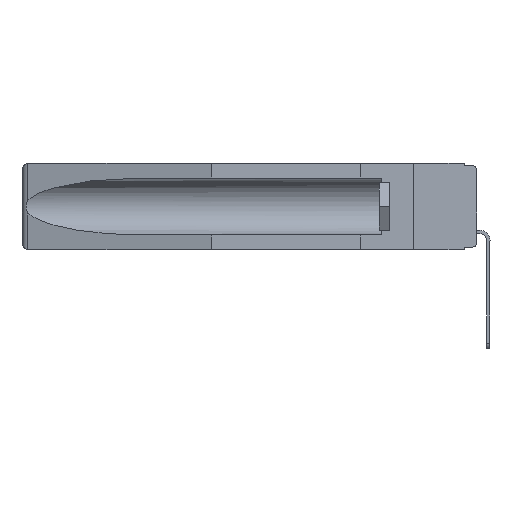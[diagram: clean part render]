
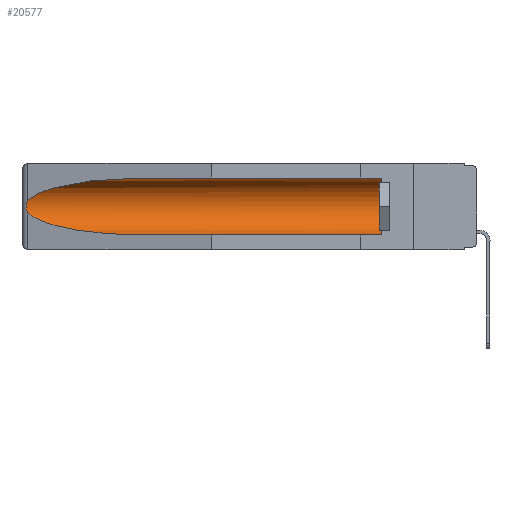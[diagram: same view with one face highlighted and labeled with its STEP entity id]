
A CAD part, left-side view. The second image highlights one B-rep face of the part: STEP entity #20577.
In plain terms, the highlighted cylindrical face has radius 2.857 mm (diameter 5.715 mm), a partial arc.
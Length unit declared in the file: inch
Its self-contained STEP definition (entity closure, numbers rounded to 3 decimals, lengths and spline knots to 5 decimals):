
#275 = CARTESIAN_POINT ( 'NONE',  ( 0.26537, 1.52718, -0.19328 ) ) ;
#886 = ORIENTED_EDGE ( 'NONE', *, *, #13939, .T. ) ;
#1474 = VECTOR ( 'NONE', #20221, 39.37008 ) ;
#1631 = CARTESIAN_POINT ( 'NONE',  ( 0.26537, 1.52718, -0.19328 ) ) ;
#1986 = VERTEX_POINT ( 'NONE', #13730 ) ;
#2005 = LINE ( 'NONE', #2962, #1474 ) ;
#2304 = FACE_OUTER_BOUND ( 'NONE', #18961, .T. ) ;
#2488 = DIRECTION ( 'NONE',  ( 0., 0., 1. ) ) ;
#2566 = CARTESIAN_POINT ( 'NONE',  ( 0.155, 0.126, -0.059 ) ) ;
#2868 = CARTESIAN_POINT ( 'NONE',  ( 0.155, 0.126, -0.284 ) ) ;
#2962 = CARTESIAN_POINT ( 'NONE',  ( 0.155, -0.30754, -0.284 ) ) ;
#3225 = CARTESIAN_POINT ( 'NONE',  ( 0.2673, 1.5327, -0.16383 ) ) ;
#4005 = VERTEX_POINT ( 'NONE', #9888 ) ;
#4371 = B_SPLINE_CURVE_WITH_KNOTS ( 'NONE', 3,
 ( #8322, #6607, #12025, #3225, #10225, #15482, #6770, #18825, #20487, #1631 ),
 .UNSPECIFIED., .F., .F.,
 ( 4, 2, 2, 2, 4 ),
 ( 0., 0.00029, 0.00058, 0.00087, 0.00117 ),
 .UNSPECIFIED. ) ;
#4438 = AXIS2_PLACEMENT_3D ( 'NONE', #12884, #14529, #2488 ) ;
#4991 = DIRECTION ( 'NONE',  ( 0., 1., 0. ) ) ;
#5295 = VERTEX_POINT ( 'NONE', #13356 ) ;
#5357 = CARTESIAN_POINT ( 'NONE',  ( 0.25451, 1.48313, -0.24835 ) ) ;
#5418 = CARTESIAN_POINT ( 'NONE',  ( 0.21114, 1.30732, -0.284 ) ) ;
#5749 =( BOUNDED_CURVE ( )  B_SPLINE_CURVE ( 3, ( #275, #5357, #5418, #10548 ),
 .UNSPECIFIED., .F., .F. ) 
 B_SPLINE_CURVE_WITH_KNOTS ( ( 4, 4 ),
 ( 0.1948, 1.5708 ),
 .UNSPECIFIED. ) 
 CURVE ( )  GEOMETRIC_REPRESENTATION_ITEM ( )  RATIONAL_B_SPLINE_CURVE ( ( 1., 0.848, 0.848, 1. ) ) 
 REPRESENTATION_ITEM ( '' )  );
#6581 = AXIS2_PLACEMENT_3D ( 'NONE', #17329, #21010, #17263 ) ;
#6607 = CARTESIAN_POINT ( 'NONE',  ( 0.26597, 1.52961, -0.15275 ) ) ;
#6770 = CARTESIAN_POINT ( 'NONE',  ( 0.2673, 1.53269, -0.17917 ) ) ;
#7017 =( BOUNDED_CURVE ( )  B_SPLINE_CURVE ( 3, ( #19918, #9661, #7828, #16526 ),
 .UNSPECIFIED., .F., .T. ) 
 B_SPLINE_CURVE_WITH_KNOTS ( ( 4, 4 ),
 ( 4.71239, 6.08839 ),
 .UNSPECIFIED. ) 
 CURVE ( )  GEOMETRIC_REPRESENTATION_ITEM ( )  RATIONAL_B_SPLINE_CURVE ( ( 1., 0.848, 0.848, 1. ) ) 
 REPRESENTATION_ITEM ( '' )  );
#7147 = ORIENTED_EDGE ( 'NONE', *, *, #9907, .T. ) ;
#7828 = CARTESIAN_POINT ( 'NONE',  ( 0.25451, 1.48313, -0.09465 ) ) ;
#8316 = VECTOR ( 'NONE', #4991, 39.37008 ) ;
#8322 = CARTESIAN_POINT ( 'NONE',  ( 0.26537, 1.52718, -0.14972 ) ) ;
#9042 = CARTESIAN_POINT ( 'NONE',  ( 0.26537, 1.52718, -0.14972 ) ) ;
#9661 = CARTESIAN_POINT ( 'NONE',  ( 0.21114, 1.30732, -0.059 ) ) ;
#9888 = CARTESIAN_POINT ( 'NONE',  ( 0.155, 1.07973, -0.059 ) ) ;
#9907 = EDGE_CURVE ( 'NONE', #22015, #4005, #12125, .T. ) ;
#10225 = CARTESIAN_POINT ( 'NONE',  ( 0.2675, 1.53308, -0.16763 ) ) ;
#10548 = CARTESIAN_POINT ( 'NONE',  ( 0.155, 1.07973, -0.284 ) ) ;
#11001 = EDGE_CURVE ( 'NONE', #11233, #5295, #2005, .T. ) ;
#11203 = ORIENTED_EDGE ( 'NONE', *, *, #16398, .T. ) ;
#11233 = VERTEX_POINT ( 'NONE', #2868 ) ;
#12025 = CARTESIAN_POINT ( 'NONE',  ( 0.26654, 1.53092, -0.15636 ) ) ;
#12125 = LINE ( 'NONE', #13794, #8316 ) ;
#12374 = EDGE_CURVE ( 'NONE', #4005, #18098, #7017, .T. ) ;
#12884 = CARTESIAN_POINT ( 'NONE',  ( 0.155, 0.126, -0.1715 ) ) ;
#13356 = CARTESIAN_POINT ( 'NONE',  ( 0.155, 1.07973, -0.284 ) ) ;
#13528 = EDGE_CURVE ( 'NONE', #11233, #22015, #17179, .T. ) ;
#13730 = CARTESIAN_POINT ( 'NONE',  ( 0.26537, 1.52718, -0.19328 ) ) ;
#13794 = CARTESIAN_POINT ( 'NONE',  ( 0.155, -0.30754, -0.059 ) ) ;
#13939 = EDGE_CURVE ( 'NONE', #18098, #1986, #4371, .T. ) ;
#14179 = ORIENTED_EDGE ( 'NONE', *, *, #13528, .T. ) ;
#14529 = DIRECTION ( 'NONE',  ( 0., -1., 0. ) ) ;
#14736 = ORIENTED_EDGE ( 'NONE', *, *, #12374, .T. ) ;
#15482 = CARTESIAN_POINT ( 'NONE',  ( 0.2675, 1.53308, -0.17534 ) ) ;
#16398 = EDGE_CURVE ( 'NONE', #1986, #5295, #5749, .T. ) ;
#16526 = CARTESIAN_POINT ( 'NONE',  ( 0.26537, 1.52718, -0.14972 ) ) ;
#17179 = CIRCLE ( 'NONE', #4438, 0.1125 ) ;
#17238 = CYLINDRICAL_SURFACE ( 'NONE', #6581, 0.1125 ) ;
#17263 = DIRECTION ( 'NONE',  ( 0., 0., 1. ) ) ;
#17329 = CARTESIAN_POINT ( 'NONE',  ( 0.155, -0.30754, -0.1715 ) ) ;
#18098 = VERTEX_POINT ( 'NONE', #9042 ) ;
#18825 = CARTESIAN_POINT ( 'NONE',  ( 0.26655, 1.53094, -0.18657 ) ) ;
#18961 = EDGE_LOOP ( 'NONE', ( #14736, #886, #11203, #21458, #14179, #7147 ) ) ;
#19918 = CARTESIAN_POINT ( 'NONE',  ( 0.155, 1.07973, -0.059 ) ) ;
#20221 = DIRECTION ( 'NONE',  ( 0., 1., 0. ) ) ;
#20487 = CARTESIAN_POINT ( 'NONE',  ( 0.26597, 1.5296, -0.19026 ) ) ;
#20577 = ADVANCED_FACE ( 'NONE', ( #2304 ), #17238, .F. ) ;
#21010 = DIRECTION ( 'NONE',  ( 0., 1., 0. ) ) ;
#21458 = ORIENTED_EDGE ( 'NONE', *, *, #11001, .F. ) ;
#22015 = VERTEX_POINT ( 'NONE', #2566 ) ;
